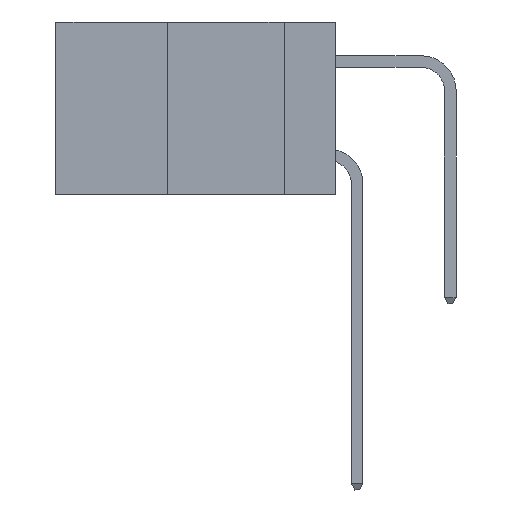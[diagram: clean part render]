
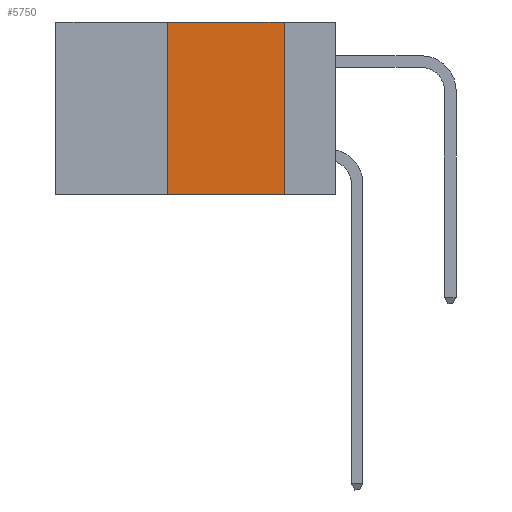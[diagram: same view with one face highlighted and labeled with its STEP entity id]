
A CAD part, left-side view. The second image highlights one B-rep face of the part: STEP entity #5750.
In plain terms, the highlighted planar face has unit normal (-1, 0, 0).
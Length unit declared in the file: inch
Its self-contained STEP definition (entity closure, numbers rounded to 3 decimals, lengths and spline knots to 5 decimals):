
#533 = AXIS2_PLACEMENT_3D ( 'NONE', #44306, #6494, #33798 ) ;
#1487 = VERTEX_POINT ( 'NONE', #11050 ) ;
#3562 = DIRECTION ( 'NONE',  ( 0., -1., 0. ) ) ;
#3679 = ORIENTED_EDGE ( 'NONE', *, *, #30214, .T. ) ;
#4446 = DIRECTION ( 'NONE',  ( 0., 0., -1. ) ) ;
#4712 = VECTOR ( 'NONE', #25325, 39.37008 ) ;
#5095 = CARTESIAN_POINT ( 'NONE',  ( 0., 0.6, 0. ) ) ;
#5283 = CARTESIAN_POINT ( 'NONE',  ( 0., 0.11, -0.37 ) ) ;
#5750 = ADVANCED_FACE ( 'NONE', ( #9730 ), #41110, .F. ) ;
#6140 = ORIENTED_EDGE ( 'NONE', *, *, #35512, .F. ) ;
#6494 = DIRECTION ( 'NONE',  ( 1., 0., 0. ) ) ;
#7084 = CARTESIAN_POINT ( 'NONE',  ( 0., 0.11, 0. ) ) ;
#8974 = VECTOR ( 'NONE', #3562, 39.37008 ) ;
#9648 = LINE ( 'NONE', #31850, #4712 ) ;
#9730 = FACE_OUTER_BOUND ( 'NONE', #16423, .T. ) ;
#10082 = LINE ( 'NONE', #34846, #8974 ) ;
#11050 = CARTESIAN_POINT ( 'NONE',  ( 0., 0.36, -0.37 ) ) ;
#15902 = VECTOR ( 'NONE', #4446, 39.37008 ) ;
#16423 = EDGE_LOOP ( 'NONE', ( #6140, #18338, #35893, #3679 ) ) ;
#16465 = LINE ( 'NONE', #21856, #15902 ) ;
#18265 = LINE ( 'NONE', #5095, #35719 ) ;
#18338 = ORIENTED_EDGE ( 'NONE', *, *, #29938, .F. ) ;
#21856 = CARTESIAN_POINT ( 'NONE',  ( 0., 0.11, 0. ) ) ;
#25325 = DIRECTION ( 'NONE',  ( 0., 0., 1. ) ) ;
#26488 = DIRECTION ( 'NONE',  ( 0., -1., 0. ) ) ;
#28335 = EDGE_CURVE ( 'NONE', #1487, #32950, #9648, .T. ) ;
#29938 = EDGE_CURVE ( 'NONE', #32950, #34495, #18265, .T. ) ;
#30214 = EDGE_CURVE ( 'NONE', #1487, #43979, #10082, .T. ) ;
#31850 = CARTESIAN_POINT ( 'NONE',  ( 0., 0.36, 0. ) ) ;
#32732 = CARTESIAN_POINT ( 'NONE',  ( 0., 0.36, 0. ) ) ;
#32950 = VERTEX_POINT ( 'NONE', #32732 ) ;
#33798 = DIRECTION ( 'NONE',  ( 0., 0., -1. ) ) ;
#34495 = VERTEX_POINT ( 'NONE', #7084 ) ;
#34846 = CARTESIAN_POINT ( 'NONE',  ( 0., 0.6, -0.37 ) ) ;
#35512 = EDGE_CURVE ( 'NONE', #34495, #43979, #16465, .T. ) ;
#35719 = VECTOR ( 'NONE', #26488, 39.37008 ) ;
#35893 = ORIENTED_EDGE ( 'NONE', *, *, #28335, .F. ) ;
#41110 = PLANE ( 'NONE',  #533 ) ;
#43979 = VERTEX_POINT ( 'NONE', #5283 ) ;
#44306 = CARTESIAN_POINT ( 'NONE',  ( 0., 0.6, 0. ) ) ;
